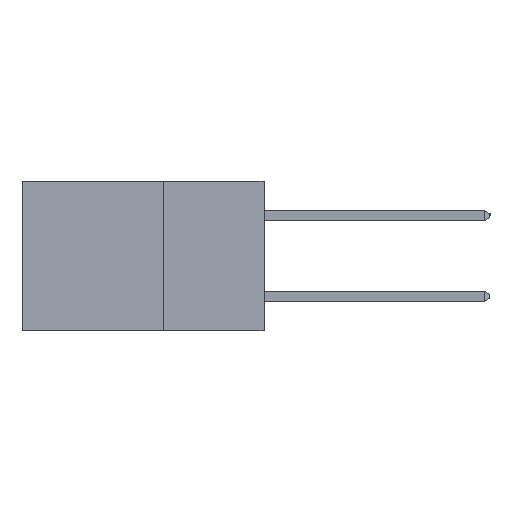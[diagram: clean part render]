
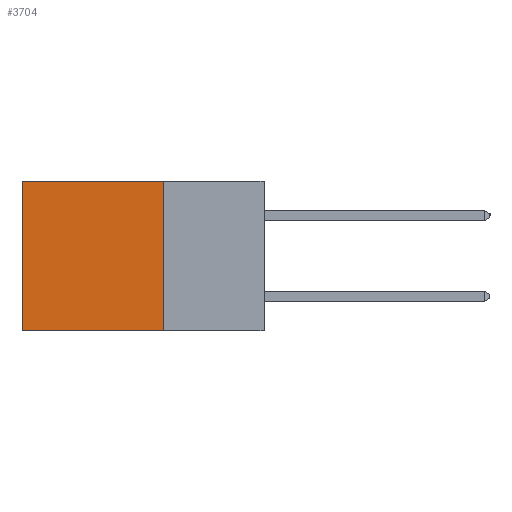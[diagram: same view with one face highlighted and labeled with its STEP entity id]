
A CAD part, left-side view. The second image highlights one B-rep face of the part: STEP entity #3704.
In plain terms, the highlighted planar face has unit normal (-1, 0, 0).
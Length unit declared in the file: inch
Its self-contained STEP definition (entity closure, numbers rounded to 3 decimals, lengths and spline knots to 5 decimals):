
#836 = VERTEX_POINT ( 'NONE', #6301 ) ;
#1575 = VECTOR ( 'NONE', #19981, 39.37008 ) ;
#2225 = FACE_OUTER_BOUND ( 'NONE', #15629, .T. ) ;
#2730 = EDGE_CURVE ( 'NONE', #13990, #19599, #6513, .T. ) ;
#2863 = CARTESIAN_POINT ( 'NONE',  ( 0.2615, 0.6, 0. ) ) ;
#3048 = CARTESIAN_POINT ( 'NONE',  ( 0.2615, 0.25, -0.37 ) ) ;
#3704 = ADVANCED_FACE ( 'NONE', ( #2225 ), #21441, .F. ) ;
#3734 = VECTOR ( 'NONE', #23085, 39.37008 ) ;
#4301 = ORIENTED_EDGE ( 'NONE', *, *, #2730, .F. ) ;
#4354 = CARTESIAN_POINT ( 'NONE',  ( 0.2615, 0.25, 0. ) ) ;
#5375 = EDGE_CURVE ( 'NONE', #836, #22349, #21317, .T. ) ;
#6301 = CARTESIAN_POINT ( 'NONE',  ( 0.2615, 0.25, 0. ) ) ;
#6430 = DIRECTION ( 'NONE',  ( 0., 0., -1. ) ) ;
#6513 = LINE ( 'NONE', #14157, #24175 ) ;
#7896 = CARTESIAN_POINT ( 'NONE',  ( 0.2615, 0.25, -0.37 ) ) ;
#10131 = CARTESIAN_POINT ( 'NONE',  ( 0.2615, 0.6, -0.37 ) ) ;
#12059 = LINE ( 'NONE', #3048, #14315 ) ;
#12385 = CARTESIAN_POINT ( 'NONE',  ( 0.2615, 0.6, -0.37 ) ) ;
#12739 = ORIENTED_EDGE ( 'NONE', *, *, #19678, .T. ) ;
#13990 = VERTEX_POINT ( 'NONE', #7896 ) ;
#14157 = CARTESIAN_POINT ( 'NONE',  ( 0.2615, 0.25, -0.37 ) ) ;
#14315 = VECTOR ( 'NONE', #6430, 39.37008 ) ;
#15629 = EDGE_LOOP ( 'NONE', ( #12739, #4301, #18768, #23906 ) ) ;
#15840 = DIRECTION ( 'NONE',  ( 0., 0., -1. ) ) ;
#17288 = EDGE_CURVE ( 'NONE', #836, #13990, #12059, .T. ) ;
#17653 = DIRECTION ( 'NONE',  ( 0., 1., 0. ) ) ;
#17906 = AXIS2_PLACEMENT_3D ( 'NONE', #21315, #19440, #15840 ) ;
#18768 = ORIENTED_EDGE ( 'NONE', *, *, #17288, .F. ) ;
#19440 = DIRECTION ( 'NONE',  ( 1., 0., 0. ) ) ;
#19599 = VERTEX_POINT ( 'NONE', #10131 ) ;
#19678 = EDGE_CURVE ( 'NONE', #22349, #19599, #21708, .T. ) ;
#19981 = DIRECTION ( 'NONE',  ( 0., 0., -1. ) ) ;
#21315 = CARTESIAN_POINT ( 'NONE',  ( 0.2615, 0.25, -0.37 ) ) ;
#21317 = LINE ( 'NONE', #4354, #3734 ) ;
#21441 = PLANE ( 'NONE',  #17906 ) ;
#21708 = LINE ( 'NONE', #12385, #1575 ) ;
#22349 = VERTEX_POINT ( 'NONE', #2863 ) ;
#23085 = DIRECTION ( 'NONE',  ( 0., 1., 0. ) ) ;
#23906 = ORIENTED_EDGE ( 'NONE', *, *, #5375, .T. ) ;
#24175 = VECTOR ( 'NONE', #17653, 39.37008 ) ;
